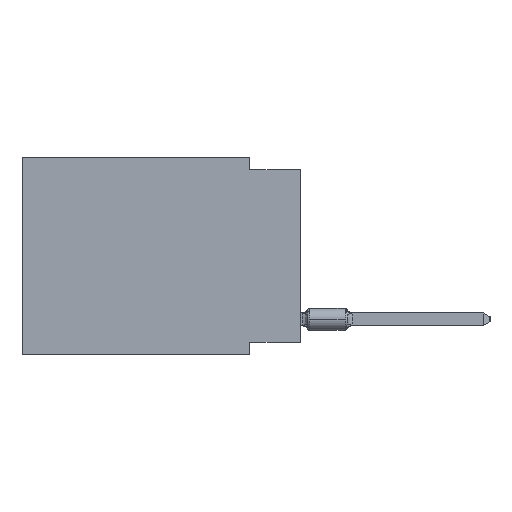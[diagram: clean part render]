
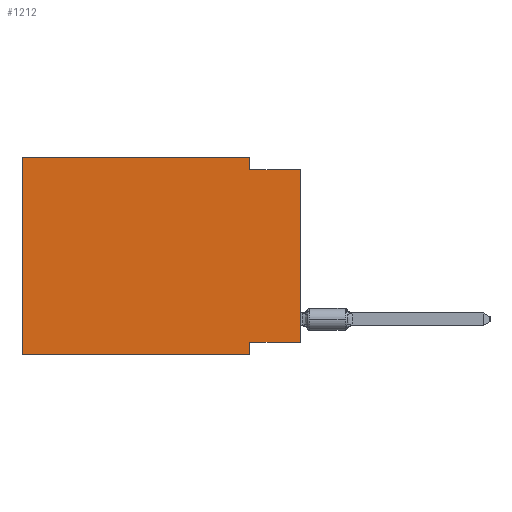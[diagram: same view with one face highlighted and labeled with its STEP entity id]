
A CAD part, left-side view. The second image highlights one B-rep face of the part: STEP entity #1212.
In plain terms, the highlighted planar face has unit normal (-1, 0, 0).
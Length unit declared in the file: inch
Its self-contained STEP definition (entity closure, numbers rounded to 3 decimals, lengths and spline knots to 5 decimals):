
#84 = CARTESIAN_POINT ( 'NONE',  ( 0., 0.1, 0. ) ) ;
#1212 = ADVANCED_FACE ( 'NONE', ( #31943 ), #2458, .F. ) ;
#1260 = DIRECTION ( 'NONE',  ( 0., 0., 1. ) ) ;
#1913 = EDGE_CURVE ( 'NONE', #27176, #24927, #42125, .T. ) ;
#2458 = PLANE ( 'NONE',  #28040 ) ;
#2915 = LINE ( 'NONE', #19377, #29651 ) ;
#4115 = CARTESIAN_POINT ( 'NONE',  ( 0., 0.55, 0. ) ) ;
#4242 = EDGE_LOOP ( 'NONE', ( #12367, #21244, #50404, #44324, #49332, #13081, #40656, #44606 ) ) ;
#4674 = VECTOR ( 'NONE', #51616, 39.37008 ) ;
#4942 = EDGE_CURVE ( 'NONE', #27176, #11573, #30202, .T. ) ;
#6398 = CARTESIAN_POINT ( 'NONE',  ( 0., 0., -0.365 ) ) ;
#7938 = LINE ( 'NONE', #47794, #22020 ) ;
#8150 = DIRECTION ( 'NONE',  ( 0., 0., 1. ) ) ;
#8548 = VERTEX_POINT ( 'NONE', #25872 ) ;
#10174 = VECTOR ( 'NONE', #46371, 39.37008 ) ;
#11565 = VERTEX_POINT ( 'NONE', #37055 ) ;
#11573 = VERTEX_POINT ( 'NONE', #4115 ) ;
#11930 = DIRECTION ( 'NONE',  ( 0., -1., 0. ) ) ;
#12367 = ORIENTED_EDGE ( 'NONE', *, *, #34990, .T. ) ;
#13081 = ORIENTED_EDGE ( 'NONE', *, *, #1913, .T. ) ;
#13596 = EDGE_CURVE ( 'NONE', #44197, #11565, #2915, .T. ) ;
#13602 = EDGE_CURVE ( 'NONE', #16008, #33005, #7938, .T. ) ;
#15927 = CARTESIAN_POINT ( 'NONE',  ( 0., 0.55, 0. ) ) ;
#16008 = VERTEX_POINT ( 'NONE', #46735 ) ;
#16445 = LINE ( 'NONE', #15927, #26873 ) ;
#17838 = VECTOR ( 'NONE', #8150, 39.37008 ) ;
#19116 = DIRECTION ( 'NONE',  ( 0., 1., 0. ) ) ;
#19193 = DIRECTION ( 'NONE',  ( 0., 0., -1. ) ) ;
#19377 = CARTESIAN_POINT ( 'NONE',  ( 0., 0., -0.365 ) ) ;
#20172 = DIRECTION ( 'NONE',  ( 0., -1., 0. ) ) ;
#20438 = VECTOR ( 'NONE', #1260, 39.37008 ) ;
#21244 = ORIENTED_EDGE ( 'NONE', *, *, #13602, .F. ) ;
#21473 = EDGE_CURVE ( 'NONE', #8548, #16008, #31969, .T. ) ;
#21635 = CARTESIAN_POINT ( 'NONE',  ( 0., 0.55, -0.39 ) ) ;
#21946 = CARTESIAN_POINT ( 'NONE',  ( 0., 0.55, -0.39 ) ) ;
#22020 = VECTOR ( 'NONE', #11930, 39.37008 ) ;
#23201 = CARTESIAN_POINT ( 'NONE',  ( 0., 0.1, -0.39 ) ) ;
#24927 = VERTEX_POINT ( 'NONE', #23201 ) ;
#25872 = CARTESIAN_POINT ( 'NONE',  ( 0., 0.1, 0. ) ) ;
#26873 = VECTOR ( 'NONE', #20172, 39.37008 ) ;
#27176 = VERTEX_POINT ( 'NONE', #21635 ) ;
#28040 = AXIS2_PLACEMENT_3D ( 'NONE', #31405, #38852, #19193 ) ;
#28349 = CARTESIAN_POINT ( 'NONE',  ( 0., 0., 0. ) ) ;
#29064 = CARTESIAN_POINT ( 'NONE',  ( 0., 0.1, -0.39 ) ) ;
#29651 = VECTOR ( 'NONE', #19116, 39.37008 ) ;
#30202 = LINE ( 'NONE', #33670, #20438 ) ;
#30484 = EDGE_CURVE ( 'NONE', #11573, #8548, #16445, .T. ) ;
#31405 = CARTESIAN_POINT ( 'NONE',  ( 0., 0.55, 0. ) ) ;
#31943 = FACE_OUTER_BOUND ( 'NONE', #4242, .T. ) ;
#31969 = LINE ( 'NONE', #84, #4674 ) ;
#32587 = EDGE_CURVE ( 'NONE', #11565, #24927, #49240, .T. ) ;
#33005 = VERTEX_POINT ( 'NONE', #49172 ) ;
#33670 = CARTESIAN_POINT ( 'NONE',  ( 0., 0.55, 0. ) ) ;
#34990 = EDGE_CURVE ( 'NONE', #44197, #33005, #48531, .T. ) ;
#37055 = CARTESIAN_POINT ( 'NONE',  ( 0., 0.1, -0.365 ) ) ;
#37220 = VECTOR ( 'NONE', #45777, 39.37008 ) ;
#38852 = DIRECTION ( 'NONE',  ( 1., 0., 0. ) ) ;
#40656 = ORIENTED_EDGE ( 'NONE', *, *, #32587, .F. ) ;
#42125 = LINE ( 'NONE', #21946, #10174 ) ;
#44197 = VERTEX_POINT ( 'NONE', #6398 ) ;
#44324 = ORIENTED_EDGE ( 'NONE', *, *, #30484, .F. ) ;
#44606 = ORIENTED_EDGE ( 'NONE', *, *, #13596, .F. ) ;
#45777 = DIRECTION ( 'NONE',  ( 0., 0., -1. ) ) ;
#46371 = DIRECTION ( 'NONE',  ( 0., -1., 0. ) ) ;
#46735 = CARTESIAN_POINT ( 'NONE',  ( 0., 0.1, -0.025 ) ) ;
#47794 = CARTESIAN_POINT ( 'NONE',  ( 0., 0., -0.025 ) ) ;
#48531 = LINE ( 'NONE', #28349, #17838 ) ;
#49172 = CARTESIAN_POINT ( 'NONE',  ( 0., 0., -0.025 ) ) ;
#49240 = LINE ( 'NONE', #29064, #37220 ) ;
#49332 = ORIENTED_EDGE ( 'NONE', *, *, #4942, .F. ) ;
#50404 = ORIENTED_EDGE ( 'NONE', *, *, #21473, .F. ) ;
#51616 = DIRECTION ( 'NONE',  ( 0., 0., -1. ) ) ;
